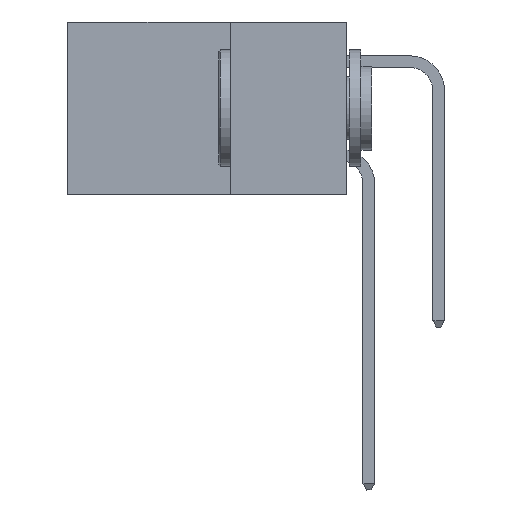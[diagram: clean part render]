
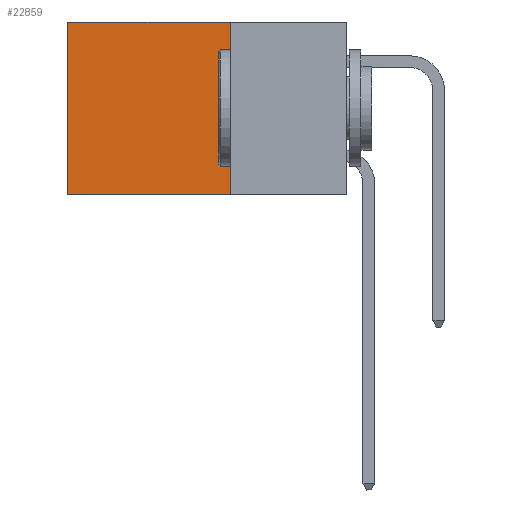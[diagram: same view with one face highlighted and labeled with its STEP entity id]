
A CAD part, left-side view. The second image highlights one B-rep face of the part: STEP entity #22859.
In plain terms, the highlighted planar face has unit normal (-1, 0, 0).
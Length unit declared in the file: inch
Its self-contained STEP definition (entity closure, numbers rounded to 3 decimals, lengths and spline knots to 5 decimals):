
#2266 = PLANE ( 'NONE',  #21039 ) ;
#4329 = ORIENTED_EDGE ( 'NONE', *, *, #5803, .T. ) ;
#4427 = VECTOR ( 'NONE', #34409, 39.37008 ) ;
#5803 = EDGE_CURVE ( 'NONE', #10655, #32742, #16650, .T. ) ;
#6851 = CARTESIAN_POINT ( 'NONE',  ( 0.2875, 0.6, -0.37 ) ) ;
#7146 = DIRECTION ( 'NONE',  ( 0., 0., -1. ) ) ;
#7236 = ORIENTED_EDGE ( 'NONE', *, *, #13434, .F. ) ;
#7917 = VERTEX_POINT ( 'NONE', #6851 ) ;
#8150 = CARTESIAN_POINT ( 'NONE',  ( 0.2875, 0.25, 0. ) ) ;
#8520 = ORIENTED_EDGE ( 'NONE', *, *, #35569, .F. ) ;
#8869 = VECTOR ( 'NONE', #23640, 39.37008 ) ;
#10655 = VERTEX_POINT ( 'NONE', #10760 ) ;
#10760 = CARTESIAN_POINT ( 'NONE',  ( 0.2875, 0.25, 0. ) ) ;
#10978 = CARTESIAN_POINT ( 'NONE',  ( 0.2875, 0.25, -0.37 ) ) ;
#11818 = LINE ( 'NONE', #13153, #20530 ) ;
#13153 = CARTESIAN_POINT ( 'NONE',  ( 0.2875, 0.6, 0. ) ) ;
#13434 = EDGE_CURVE ( 'NONE', #10655, #31346, #33100, .T. ) ;
#14027 = DIRECTION ( 'NONE',  ( 0., 0., -1. ) ) ;
#14794 = CARTESIAN_POINT ( 'NONE',  ( 0.2875, 0.25, 0. ) ) ;
#16650 = LINE ( 'NONE', #14794, #8869 ) ;
#18190 = CARTESIAN_POINT ( 'NONE',  ( 0.2875, 0.25, -0.37 ) ) ;
#18977 = CARTESIAN_POINT ( 'NONE',  ( 0.2875, 0.6, 0. ) ) ;
#20530 = VECTOR ( 'NONE', #7146, 39.37008 ) ;
#20838 = DIRECTION ( 'NONE',  ( 0., 0., -1. ) ) ;
#21039 = AXIS2_PLACEMENT_3D ( 'NONE', #8150, #31606, #14027 ) ;
#22859 = ADVANCED_FACE ( 'NONE', ( #27921 ), #2266, .F. ) ;
#23640 = DIRECTION ( 'NONE',  ( 0., 1., 0. ) ) ;
#24940 = EDGE_LOOP ( 'NONE', ( #28529, #8520, #7236, #4329 ) ) ;
#25295 = VECTOR ( 'NONE', #20838, 39.37008 ) ;
#27921 = FACE_OUTER_BOUND ( 'NONE', #24940, .T. ) ;
#28529 = ORIENTED_EDGE ( 'NONE', *, *, #30200, .T. ) ;
#30200 = EDGE_CURVE ( 'NONE', #32742, #7917, #11818, .T. ) ;
#31346 = VERTEX_POINT ( 'NONE', #18190 ) ;
#31606 = DIRECTION ( 'NONE',  ( 1., 0., 0. ) ) ;
#32525 = CARTESIAN_POINT ( 'NONE',  ( 0.2875, 0.25, 0. ) ) ;
#32742 = VERTEX_POINT ( 'NONE', #18977 ) ;
#33100 = LINE ( 'NONE', #32525, #25295 ) ;
#34409 = DIRECTION ( 'NONE',  ( 0., 1., 0. ) ) ;
#34628 = LINE ( 'NONE', #10978, #4427 ) ;
#35569 = EDGE_CURVE ( 'NONE', #31346, #7917, #34628, .T. ) ;
